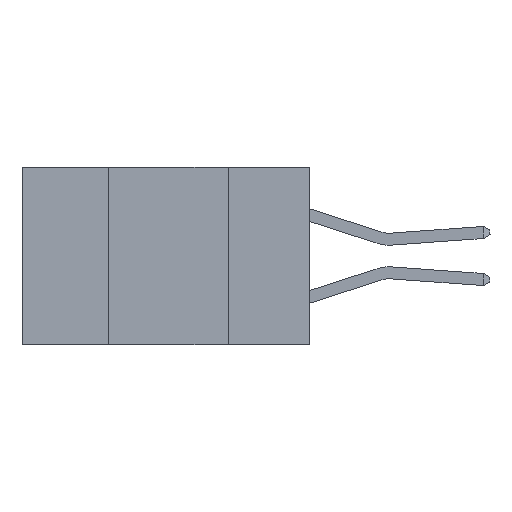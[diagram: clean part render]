
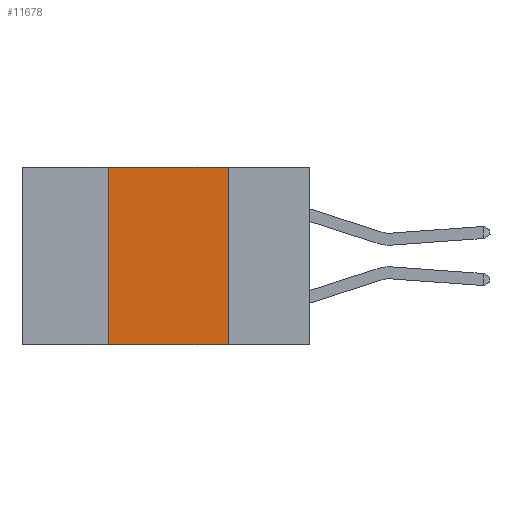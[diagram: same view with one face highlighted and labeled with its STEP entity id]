
A CAD part, left-side view. The second image highlights one B-rep face of the part: STEP entity #11678.
In plain terms, the highlighted planar face has unit normal (-1, 0, 0).
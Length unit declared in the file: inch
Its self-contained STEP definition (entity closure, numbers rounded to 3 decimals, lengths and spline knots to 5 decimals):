
#326 = EDGE_CURVE ( 'NONE', #17472, #14045, #5374, .T. ) ;
#1424 = CARTESIAN_POINT ( 'NONE',  ( 0., 0.17, 0. ) ) ;
#2129 = CARTESIAN_POINT ( 'NONE',  ( 0., 0.42, 0. ) ) ;
#2691 = EDGE_CURVE ( 'NONE', #17425, #4649, #4306, .T. ) ;
#3037 = LINE ( 'NONE', #3595, #12704 ) ;
#3595 = CARTESIAN_POINT ( 'NONE',  ( 0., 0.6, 0. ) ) ;
#4306 = LINE ( 'NONE', #9649, #17388 ) ;
#4649 = VERTEX_POINT ( 'NONE', #4822 ) ;
#4822 = CARTESIAN_POINT ( 'NONE',  ( 0., 0.17, -0.37 ) ) ;
#5374 = LINE ( 'NONE', #2129, #7066 ) ;
#5823 = EDGE_LOOP ( 'NONE', ( #16818, #7356, #16232, #13021 ) ) ;
#6635 = AXIS2_PLACEMENT_3D ( 'NONE', #13237, #15909, #7665 ) ;
#6893 = EDGE_CURVE ( 'NONE', #17472, #4649, #13573, .T. ) ;
#7066 = VECTOR ( 'NONE', #12912, 39.37008 ) ;
#7170 = EDGE_CURVE ( 'NONE', #14045, #17425, #3037, .T. ) ;
#7356 = ORIENTED_EDGE ( 'NONE', *, *, #7170, .F. ) ;
#7665 = DIRECTION ( 'NONE',  ( 0., 0., -1. ) ) ;
#9198 = CARTESIAN_POINT ( 'NONE',  ( 0., 0.42, -0.37 ) ) ;
#9285 = DIRECTION ( 'NONE',  ( 0., -1., 0. ) ) ;
#9379 = FACE_OUTER_BOUND ( 'NONE', #5823, .T. ) ;
#9649 = CARTESIAN_POINT ( 'NONE',  ( 0., 0.17, 0. ) ) ;
#10972 = CARTESIAN_POINT ( 'NONE',  ( 0., 0.42, 0. ) ) ;
#11428 = VECTOR ( 'NONE', #9285, 39.37008 ) ;
#11678 = ADVANCED_FACE ( 'NONE', ( #9379 ), #17169, .F. ) ;
#12413 = DIRECTION ( 'NONE',  ( 0., 0., -1. ) ) ;
#12704 = VECTOR ( 'NONE', #14425, 39.37008 ) ;
#12912 = DIRECTION ( 'NONE',  ( 0., 0., 1. ) ) ;
#13021 = ORIENTED_EDGE ( 'NONE', *, *, #6893, .T. ) ;
#13237 = CARTESIAN_POINT ( 'NONE',  ( 0., 0.6, 0. ) ) ;
#13573 = LINE ( 'NONE', #16143, #11428 ) ;
#14045 = VERTEX_POINT ( 'NONE', #10972 ) ;
#14425 = DIRECTION ( 'NONE',  ( 0., -1., 0. ) ) ;
#15909 = DIRECTION ( 'NONE',  ( 1., 0., 0. ) ) ;
#16143 = CARTESIAN_POINT ( 'NONE',  ( 0., 0.6, -0.37 ) ) ;
#16232 = ORIENTED_EDGE ( 'NONE', *, *, #326, .F. ) ;
#16818 = ORIENTED_EDGE ( 'NONE', *, *, #2691, .F. ) ;
#17169 = PLANE ( 'NONE',  #6635 ) ;
#17388 = VECTOR ( 'NONE', #12413, 39.37008 ) ;
#17425 = VERTEX_POINT ( 'NONE', #1424 ) ;
#17472 = VERTEX_POINT ( 'NONE', #9198 ) ;
